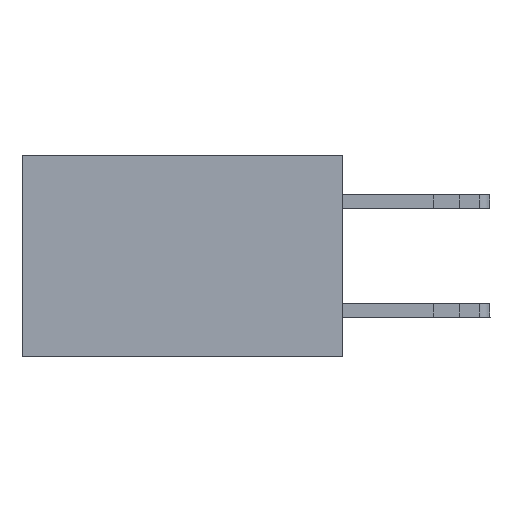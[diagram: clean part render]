
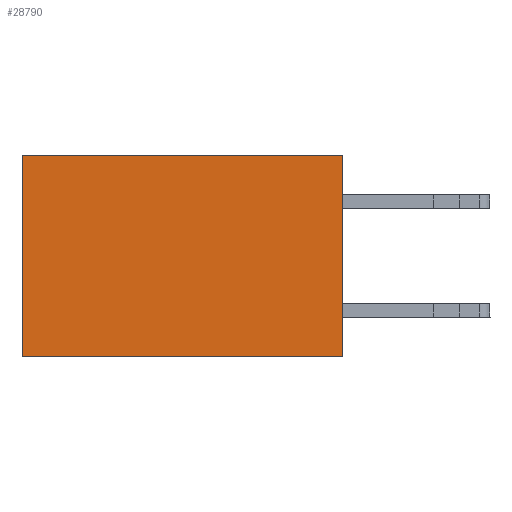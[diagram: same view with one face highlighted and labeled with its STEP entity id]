
A CAD part, left-side view. The second image highlights one B-rep face of the part: STEP entity #28790.
In plain terms, the highlighted planar face has unit normal (-1, 0, 0).
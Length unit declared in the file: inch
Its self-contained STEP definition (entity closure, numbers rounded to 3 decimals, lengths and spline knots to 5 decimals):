
#3483 = VERTEX_POINT ( 'NONE', #18991 ) ;
#3852 = PLANE ( 'NONE',  #27341 ) ;
#4735 = VERTEX_POINT ( 'NONE', #20057 ) ;
#5498 = VERTEX_POINT ( 'NONE', #10831 ) ;
#6156 = DIRECTION ( 'NONE',  ( 1., 0., 0. ) ) ;
#6596 = VERTEX_POINT ( 'NONE', #10799 ) ;
#7235 = EDGE_CURVE ( 'NONE', #5498, #6596, #25084, .T. ) ;
#7693 = EDGE_CURVE ( 'NONE', #3483, #5498, #13962, .T. ) ;
#8803 = CARTESIAN_POINT ( 'NONE',  ( 0.277, 0., 0. ) ) ;
#10799 = CARTESIAN_POINT ( 'NONE',  ( 0.277, 0.59, -0.37 ) ) ;
#10831 = CARTESIAN_POINT ( 'NONE',  ( 0.277, 0., -0.37 ) ) ;
#12647 = EDGE_CURVE ( 'NONE', #3483, #4735, #19160, .T. ) ;
#13962 = LINE ( 'NONE', #15102, #19196 ) ;
#14185 = LINE ( 'NONE', #19677, #19431 ) ;
#14928 = ORIENTED_EDGE ( 'NONE', *, *, #7235, .F. ) ;
#15059 = ORIENTED_EDGE ( 'NONE', *, *, #12647, .T. ) ;
#15102 = CARTESIAN_POINT ( 'NONE',  ( 0.277, 0., -0.37 ) ) ;
#15175 = DIRECTION ( 'NONE',  ( 0., 0., -1. ) ) ;
#15201 = ORIENTED_EDGE ( 'NONE', *, *, #7693, .F. ) ;
#15392 = DIRECTION ( 'NONE',  ( 0., 0., -1. ) ) ;
#16016 = EDGE_LOOP ( 'NONE', ( #23976, #14928, #15201, #15059 ) ) ;
#18991 = CARTESIAN_POINT ( 'NONE',  ( 0.277, 0., 0. ) ) ;
#19160 = LINE ( 'NONE', #8803, #24356 ) ;
#19196 = VECTOR ( 'NONE', #15392, 39.37008 ) ;
#19230 = VECTOR ( 'NONE', #26866, 39.37008 ) ;
#19431 = VECTOR ( 'NONE', #15175, 39.37008 ) ;
#19677 = CARTESIAN_POINT ( 'NONE',  ( 0.277, 0.59, -0.37 ) ) ;
#19731 = CARTESIAN_POINT ( 'NONE',  ( 0.277, 0., -0.37 ) ) ;
#20057 = CARTESIAN_POINT ( 'NONE',  ( 0.277, 0.59, 0. ) ) ;
#21682 = FACE_OUTER_BOUND ( 'NONE', #16016, .T. ) ;
#21938 = DIRECTION ( 'NONE',  ( 0., 0., -1. ) ) ;
#23976 = ORIENTED_EDGE ( 'NONE', *, *, #25273, .T. ) ;
#24356 = VECTOR ( 'NONE', #26701, 39.37008 ) ;
#25084 = LINE ( 'NONE', #26774, #19230 ) ;
#25273 = EDGE_CURVE ( 'NONE', #4735, #6596, #14185, .T. ) ;
#26701 = DIRECTION ( 'NONE',  ( 0., 1., 0. ) ) ;
#26774 = CARTESIAN_POINT ( 'NONE',  ( 0.277, 0., -0.37 ) ) ;
#26866 = DIRECTION ( 'NONE',  ( 0., 1., 0. ) ) ;
#27341 = AXIS2_PLACEMENT_3D ( 'NONE', #19731, #6156, #21938 ) ;
#28790 = ADVANCED_FACE ( 'NONE', ( #21682 ), #3852, .F. ) ;
